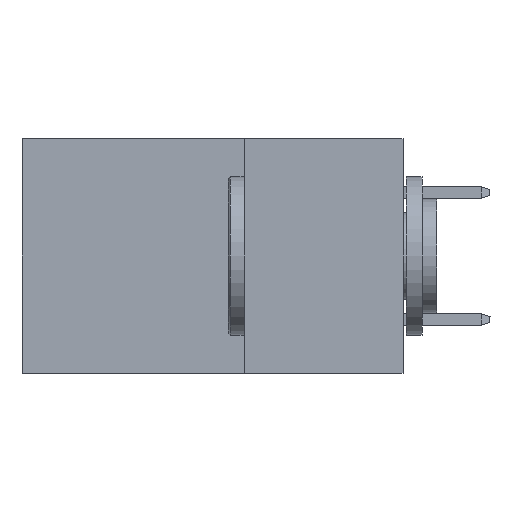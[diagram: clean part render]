
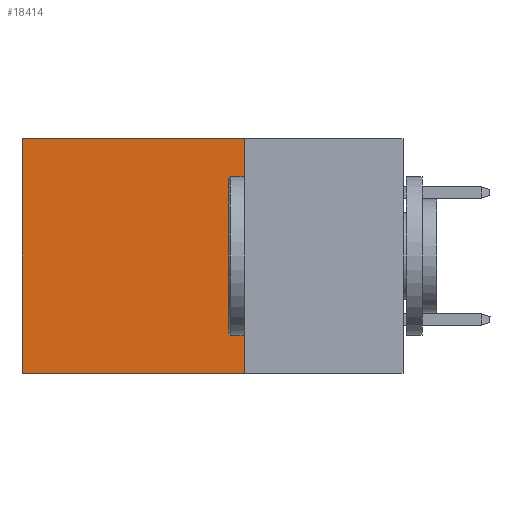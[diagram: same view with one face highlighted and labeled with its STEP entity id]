
A CAD part, left-side view. The second image highlights one B-rep face of the part: STEP entity #18414.
In plain terms, the highlighted planar face has unit normal (-1, 0, 0).
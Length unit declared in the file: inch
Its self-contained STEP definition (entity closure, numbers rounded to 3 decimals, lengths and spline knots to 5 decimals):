
#380 = DIRECTION ( 'NONE',  ( 0., 0., -1. ) ) ;
#2114 = CARTESIAN_POINT ( 'NONE',  ( 0.2875, 0.25, 0. ) ) ;
#2758 = DIRECTION ( 'NONE',  ( 0., 0., -1. ) ) ;
#3604 = EDGE_CURVE ( 'NONE', #14853, #19573, #15432, .T. ) ;
#3705 = DIRECTION ( 'NONE',  ( 0., 0., -1. ) ) ;
#4067 = CARTESIAN_POINT ( 'NONE',  ( 0.2875, 0.25, -0.37 ) ) ;
#4732 = VERTEX_POINT ( 'NONE', #11032 ) ;
#4974 = ORIENTED_EDGE ( 'NONE', *, *, #14653, .F. ) ;
#6439 = LINE ( 'NONE', #15828, #9677 ) ;
#7404 = CARTESIAN_POINT ( 'NONE',  ( 0.2875, 0.25, -0.37 ) ) ;
#7425 = VECTOR ( 'NONE', #3705, 39.37008 ) ;
#7804 = DIRECTION ( 'NONE',  ( 1., 0., 0. ) ) ;
#7901 = PLANE ( 'NONE',  #10998 ) ;
#8126 = VECTOR ( 'NONE', #2758, 39.37008 ) ;
#8240 = VERTEX_POINT ( 'NONE', #4067 ) ;
#9006 = FACE_OUTER_BOUND ( 'NONE', #17817, .T. ) ;
#9477 = DIRECTION ( 'NONE',  ( 0., 1., 0. ) ) ;
#9677 = VECTOR ( 'NONE', #9477, 39.37008 ) ;
#10375 = ORIENTED_EDGE ( 'NONE', *, *, #3604, .T. ) ;
#10811 = DIRECTION ( 'NONE',  ( 0., 1., 0. ) ) ;
#10980 = ORIENTED_EDGE ( 'NONE', *, *, #15739, .T. ) ;
#10998 = AXIS2_PLACEMENT_3D ( 'NONE', #15468, #7804, #380 ) ;
#11032 = CARTESIAN_POINT ( 'NONE',  ( 0.2875, 0.25, 0. ) ) ;
#11056 = ORIENTED_EDGE ( 'NONE', *, *, #18321, .F. ) ;
#12857 = CARTESIAN_POINT ( 'NONE',  ( 0.2875, 0.6, -0.37 ) ) ;
#14653 = EDGE_CURVE ( 'NONE', #4732, #8240, #19070, .T. ) ;
#14853 = VERTEX_POINT ( 'NONE', #18782 ) ;
#15175 = LINE ( 'NONE', #7404, #19781 ) ;
#15240 = CARTESIAN_POINT ( 'NONE',  ( 0.2875, 0.6, 0. ) ) ;
#15432 = LINE ( 'NONE', #15240, #8126 ) ;
#15468 = CARTESIAN_POINT ( 'NONE',  ( 0.2875, 0.25, 0. ) ) ;
#15739 = EDGE_CURVE ( 'NONE', #4732, #14853, #6439, .T. ) ;
#15828 = CARTESIAN_POINT ( 'NONE',  ( 0.2875, 0.25, 0. ) ) ;
#17817 = EDGE_LOOP ( 'NONE', ( #10375, #11056, #4974, #10980 ) ) ;
#18321 = EDGE_CURVE ( 'NONE', #8240, #19573, #15175, .T. ) ;
#18414 = ADVANCED_FACE ( 'NONE', ( #9006 ), #7901, .F. ) ;
#18782 = CARTESIAN_POINT ( 'NONE',  ( 0.2875, 0.6, 0. ) ) ;
#19070 = LINE ( 'NONE', #2114, #7425 ) ;
#19573 = VERTEX_POINT ( 'NONE', #12857 ) ;
#19781 = VECTOR ( 'NONE', #10811, 39.37008 ) ;
